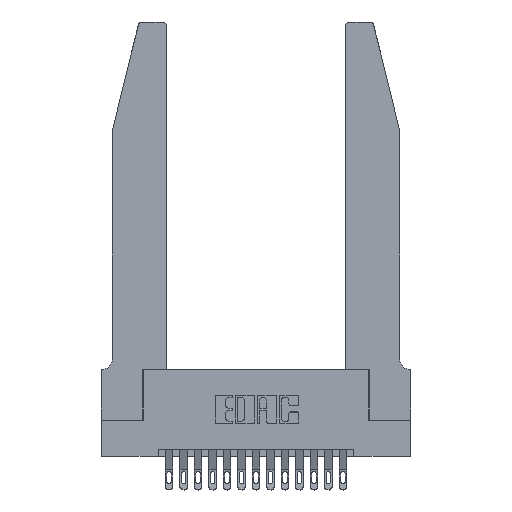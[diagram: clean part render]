
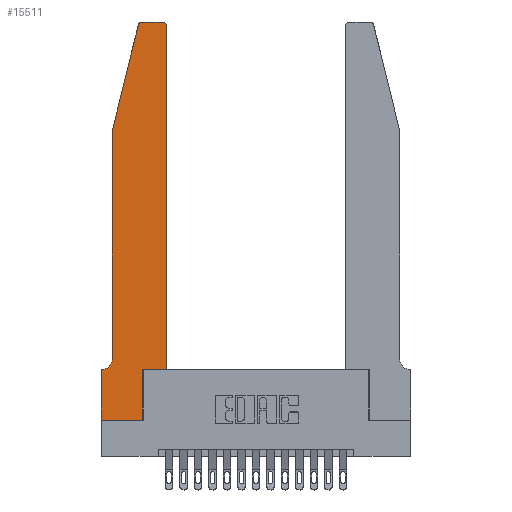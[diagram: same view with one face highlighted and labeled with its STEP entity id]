
A CAD part, top view. The second image highlights one B-rep face of the part: STEP entity #15511.
In plain terms, the highlighted planar face has unit normal (0, 0, 1).
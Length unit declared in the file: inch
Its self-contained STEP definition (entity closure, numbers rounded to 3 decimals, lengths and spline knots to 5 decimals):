
#5 = CARTESIAN_POINT ( 'NONE',  ( 0., 0., 0.37 ) ) ;
#229 = EDGE_CURVE ( 'NONE', #5733, #9988, #15879, .T. ) ;
#241 = ORIENTED_EDGE ( 'NONE', *, *, #6842, .T. ) ;
#794 = VECTOR ( 'NONE', #15103, 39.37008 ) ;
#1076 = VERTEX_POINT ( 'NONE', #15893 ) ;
#1089 = DIRECTION ( 'NONE',  ( 0., 0., 1. ) ) ;
#1233 = DIRECTION ( 'NONE',  ( 0., 0., -1. ) ) ;
#1416 = DIRECTION ( 'NONE',  ( -1., 0., 0. ) ) ;
#1469 = DIRECTION ( 'NONE',  ( 0., 1., 0. ) ) ;
#1551 = CARTESIAN_POINT ( 'NONE',  ( 0.2865, 0., 0.37 ) ) ;
#1573 = LINE ( 'NONE', #17837, #16850 ) ;
#1629 = ORIENTED_EDGE ( 'NONE', *, *, #13555, .T. ) ;
#1979 = EDGE_CURVE ( 'NONE', #2537, #15857, #9261, .T. ) ;
#2228 = VERTEX_POINT ( 'NONE', #16989 ) ;
#2490 = CARTESIAN_POINT ( 'NONE',  ( 0., 0., 0.37 ) ) ;
#2537 = VERTEX_POINT ( 'NONE', #1551 ) ;
#3521 = ORIENTED_EDGE ( 'NONE', *, *, #229, .T. ) ;
#3536 = EDGE_CURVE ( 'NONE', #17486, #15794, #14332, .T. ) ;
#3616 = LINE ( 'NONE', #9141, #5252 ) ;
#3681 = DIRECTION ( 'NONE',  ( 0., -1., 0. ) ) ;
#3742 = VECTOR ( 'NONE', #17452, 39.37008 ) ;
#4064 = LINE ( 'NONE', #14343, #4530 ) ;
#4160 = CARTESIAN_POINT ( 'NONE',  ( 0.284, 2.72, 0.37 ) ) ;
#4174 = CARTESIAN_POINT ( 'NONE',  ( 0.25487, 2.72718, 0.37 ) ) ;
#4337 = CARTESIAN_POINT ( 'NONE',  ( 0., 0., 0.37 ) ) ;
#4530 = VECTOR ( 'NONE', #17457, 39.37008 ) ;
#4561 = DIRECTION ( 'NONE',  ( -1., 0., 0. ) ) ;
#4696 = LINE ( 'NONE', #13684, #794 ) ;
#4830 = VECTOR ( 'NONE', #13225, 39.37008 ) ;
#4880 = EDGE_CURVE ( 'NONE', #15794, #2537, #11719, .T. ) ;
#5203 = AXIS2_PLACEMENT_3D ( 'NONE', #4160, #1089, #12857 ) ;
#5252 = VECTOR ( 'NONE', #3681, 39.37008 ) ;
#5733 = VERTEX_POINT ( 'NONE', #14911 ) ;
#5833 = DIRECTION ( 'NONE',  ( 1., 0., 0. ) ) ;
#5869 = CARTESIAN_POINT ( 'NONE',  ( 0.0755, 2., 0.37 ) ) ;
#6025 = PLANE ( 'NONE',  #8111 ) ;
#6087 = EDGE_CURVE ( 'NONE', #6429, #7409, #3616, .T. ) ;
#6285 = CIRCLE ( 'NONE', #5203, 0.03 ) ;
#6429 = VERTEX_POINT ( 'NONE', #5869 ) ;
#6815 = ORIENTED_EDGE ( 'NONE', *, *, #3536, .T. ) ;
#6842 = EDGE_CURVE ( 'NONE', #9988, #1076, #15203, .T. ) ;
#7106 = CARTESIAN_POINT ( 'NONE',  ( 0.0755, 0.35, 0.37 ) ) ;
#7409 = VERTEX_POINT ( 'NONE', #8845 ) ;
#7648 = CARTESIAN_POINT ( 'NONE',  ( 0., 0.35, 0.37 ) ) ;
#7691 = LINE ( 'NONE', #7106, #3742 ) ;
#7785 = ORIENTED_EDGE ( 'NONE', *, *, #17448, .T. ) ;
#8111 = AXIS2_PLACEMENT_3D ( 'NONE', #7648, #9104, #16391 ) ;
#8256 = EDGE_LOOP ( 'NONE', ( #13774, #12718, #16971, #17465, #1629, #13527, #6815, #9116, #12011, #7785, #3521, #241 ) ) ;
#8488 = VERTEX_POINT ( 'NONE', #10443 ) ;
#8845 = CARTESIAN_POINT ( 'NONE',  ( 0.0755, 0.42, 0.37 ) ) ;
#8847 = EDGE_CURVE ( 'NONE', #14607, #6429, #4696, .T. ) ;
#8848 = CIRCLE ( 'NONE', #11013, 0.07 ) ;
#9104 = DIRECTION ( 'NONE',  ( 0., 0., 1. ) ) ;
#9116 = ORIENTED_EDGE ( 'NONE', *, *, #4880, .T. ) ;
#9124 = CARTESIAN_POINT ( 'NONE',  ( 0.2865, 0.35, 0.37 ) ) ;
#9141 = CARTESIAN_POINT ( 'NONE',  ( 0.0755, 2., 0.37 ) ) ;
#9261 = LINE ( 'NONE', #9124, #13663 ) ;
#9464 = CARTESIAN_POINT ( 'NONE',  ( 0.4505, 0.35, 0.37 ) ) ;
#9897 = EDGE_CURVE ( 'NONE', #8488, #14607, #6285, .T. ) ;
#9988 = VERTEX_POINT ( 'NONE', #14720 ) ;
#10225 = CARTESIAN_POINT ( 'NONE',  ( 0.0055, 0.42, 0.37 ) ) ;
#10443 = CARTESIAN_POINT ( 'NONE',  ( 0.284, 2.75, 0.37 ) ) ;
#11013 = AXIS2_PLACEMENT_3D ( 'NONE', #10225, #1233, #1416 ) ;
#11404 = CARTESIAN_POINT ( 'NONE',  ( 0.4205, 2.72, 0.37 ) ) ;
#11461 = CARTESIAN_POINT ( 'NONE',  ( 0.2865, 0.35, 0.37 ) ) ;
#11719 = LINE ( 'NONE', #4337, #12171 ) ;
#12011 = ORIENTED_EDGE ( 'NONE', *, *, #1979, .T. ) ;
#12171 = VECTOR ( 'NONE', #5833, 39.37008 ) ;
#12267 = DIRECTION ( 'NONE',  ( 0., 1., 0. ) ) ;
#12718 = ORIENTED_EDGE ( 'NONE', *, *, #9897, .T. ) ;
#12857 = DIRECTION ( 'NONE',  ( 1., 0., 0. ) ) ;
#13225 = DIRECTION ( 'NONE',  ( 0., -1., 0. ) ) ;
#13527 = ORIENTED_EDGE ( 'NONE', *, *, #13886, .T. ) ;
#13555 = EDGE_CURVE ( 'NONE', #7409, #2228, #8848, .T. ) ;
#13663 = VECTOR ( 'NONE', #1469, 39.37008 ) ;
#13684 = CARTESIAN_POINT ( 'NONE',  ( 0.0755, 2., 0.37 ) ) ;
#13774 = ORIENTED_EDGE ( 'NONE', *, *, #16567, .T. ) ;
#13886 = EDGE_CURVE ( 'NONE', #2228, #17486, #7691, .T. ) ;
#14332 = LINE ( 'NONE', #5, #4830 ) ;
#14343 = CARTESIAN_POINT ( 'NONE',  ( 0.4505, 0.35, 0.37 ) ) ;
#14607 = VERTEX_POINT ( 'NONE', #4174 ) ;
#14720 = CARTESIAN_POINT ( 'NONE',  ( 0.4505, 2.72, 0.37 ) ) ;
#14911 = CARTESIAN_POINT ( 'NONE',  ( 0.4505, 0.35, 0.37 ) ) ;
#15103 = DIRECTION ( 'NONE',  ( -0.239, -0.971, 0. ) ) ;
#15203 = CIRCLE ( 'NONE', #17445, 0.03 ) ;
#15511 = ADVANCED_FACE ( 'NONE', ( #15754 ), #6025, .T. ) ;
#15641 = VECTOR ( 'NONE', #12267, 39.37008 ) ;
#15754 = FACE_OUTER_BOUND ( 'NONE', #8256, .T. ) ;
#15794 = VERTEX_POINT ( 'NONE', #2490 ) ;
#15819 = DIRECTION ( 'NONE',  ( 1., 0., 0. ) ) ;
#15857 = VERTEX_POINT ( 'NONE', #11461 ) ;
#15879 = LINE ( 'NONE', #9464, #15641 ) ;
#15893 = CARTESIAN_POINT ( 'NONE',  ( 0.4205, 2.75, 0.37 ) ) ;
#16391 = DIRECTION ( 'NONE',  ( 1., 0., 0. ) ) ;
#16567 = EDGE_CURVE ( 'NONE', #1076, #8488, #1573, .T. ) ;
#16850 = VECTOR ( 'NONE', #4561, 39.37008 ) ;
#16971 = ORIENTED_EDGE ( 'NONE', *, *, #8847, .T. ) ;
#16989 = CARTESIAN_POINT ( 'NONE',  ( 0.0055, 0.35, 0.37 ) ) ;
#17202 = CARTESIAN_POINT ( 'NONE',  ( 0., 0.35, 0.37 ) ) ;
#17348 = DIRECTION ( 'NONE',  ( 0., 0., 1. ) ) ;
#17445 = AXIS2_PLACEMENT_3D ( 'NONE', #11404, #17348, #15819 ) ;
#17448 = EDGE_CURVE ( 'NONE', #15857, #5733, #4064, .T. ) ;
#17452 = DIRECTION ( 'NONE',  ( -1., 0., 0. ) ) ;
#17457 = DIRECTION ( 'NONE',  ( 1., 0., 0. ) ) ;
#17465 = ORIENTED_EDGE ( 'NONE', *, *, #6087, .T. ) ;
#17486 = VERTEX_POINT ( 'NONE', #17202 ) ;
#17837 = CARTESIAN_POINT ( 'NONE',  ( 0.2605, 2.75, 0.37 ) ) ;
